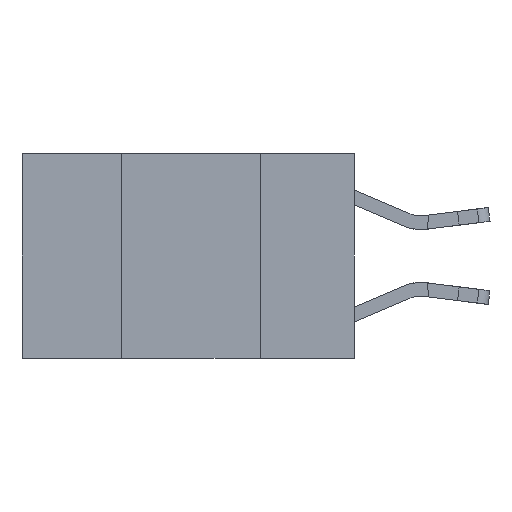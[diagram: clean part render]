
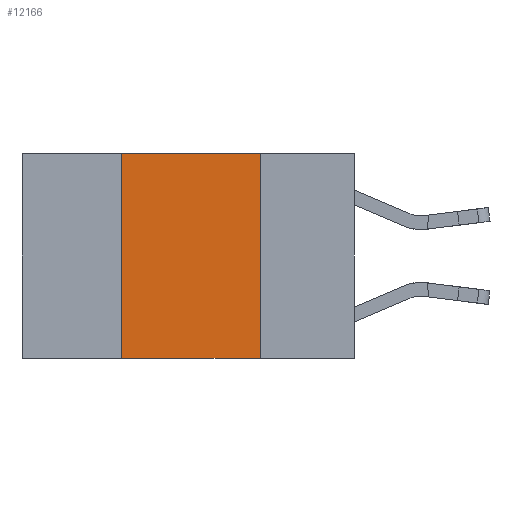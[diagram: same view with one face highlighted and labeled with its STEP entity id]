
A CAD part, left-side view. The second image highlights one B-rep face of the part: STEP entity #12166.
In plain terms, the highlighted planar face has unit normal (-1, 0, 0).
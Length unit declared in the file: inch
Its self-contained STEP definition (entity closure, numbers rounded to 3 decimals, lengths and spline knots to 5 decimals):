
#461 = EDGE_CURVE ( 'NONE', #20205, #12961, #18136, .T. ) ;
#525 = VECTOR ( 'NONE', #20339, 39.37008 ) ;
#1005 = CARTESIAN_POINT ( 'NONE',  ( 0., 0.17, -0.37 ) ) ;
#1347 = ORIENTED_EDGE ( 'NONE', *, *, #8462, .F. ) ;
#2122 = PLANE ( 'NONE',  #2619 ) ;
#2191 = DIRECTION ( 'NONE',  ( 0., 0., -1. ) ) ;
#2619 = AXIS2_PLACEMENT_3D ( 'NONE', #19766, #11817, #2191 ) ;
#3172 = LINE ( 'NONE', #17281, #19174 ) ;
#5739 = ORIENTED_EDGE ( 'NONE', *, *, #13558, .F. ) ;
#7451 = VERTEX_POINT ( 'NONE', #18464 ) ;
#7615 = EDGE_LOOP ( 'NONE', ( #1347, #5739, #14705, #19930 ) ) ;
#7695 = CARTESIAN_POINT ( 'NONE',  ( 0., 0.6, 0. ) ) ;
#8462 = EDGE_CURVE ( 'NONE', #16756, #12961, #13163, .T. ) ;
#8586 = CARTESIAN_POINT ( 'NONE',  ( 0., 0.17, 0. ) ) ;
#9190 = CARTESIAN_POINT ( 'NONE',  ( 0., 0.6, -0.37 ) ) ;
#9269 = DIRECTION ( 'NONE',  ( 0., -1., 0. ) ) ;
#11817 = DIRECTION ( 'NONE',  ( 1., 0., 0. ) ) ;
#12166 = ADVANCED_FACE ( 'NONE', ( #15539 ), #2122, .F. ) ;
#12586 = DIRECTION ( 'NONE',  ( 0., 0., 1. ) ) ;
#12643 = VECTOR ( 'NONE', #14460, 39.37008 ) ;
#12961 = VERTEX_POINT ( 'NONE', #1005 ) ;
#13037 = LINE ( 'NONE', #7695, #20511 ) ;
#13163 = LINE ( 'NONE', #16068, #12643 ) ;
#13558 = EDGE_CURVE ( 'NONE', #7451, #16756, #13037, .T. ) ;
#14460 = DIRECTION ( 'NONE',  ( 0., 0., -1. ) ) ;
#14705 = ORIENTED_EDGE ( 'NONE', *, *, #15738, .F. ) ;
#15539 = FACE_OUTER_BOUND ( 'NONE', #7615, .T. ) ;
#15738 = EDGE_CURVE ( 'NONE', #20205, #7451, #3172, .T. ) ;
#16068 = CARTESIAN_POINT ( 'NONE',  ( 0., 0.17, 0. ) ) ;
#16756 = VERTEX_POINT ( 'NONE', #8586 ) ;
#17281 = CARTESIAN_POINT ( 'NONE',  ( 0., 0.42, 0. ) ) ;
#18136 = LINE ( 'NONE', #9190, #525 ) ;
#18464 = CARTESIAN_POINT ( 'NONE',  ( 0., 0.42, 0. ) ) ;
#19174 = VECTOR ( 'NONE', #12586, 39.37008 ) ;
#19298 = CARTESIAN_POINT ( 'NONE',  ( 0., 0.42, -0.37 ) ) ;
#19766 = CARTESIAN_POINT ( 'NONE',  ( 0., 0.6, 0. ) ) ;
#19930 = ORIENTED_EDGE ( 'NONE', *, *, #461, .T. ) ;
#20205 = VERTEX_POINT ( 'NONE', #19298 ) ;
#20339 = DIRECTION ( 'NONE',  ( 0., -1., 0. ) ) ;
#20511 = VECTOR ( 'NONE', #9269, 39.37008 ) ;
